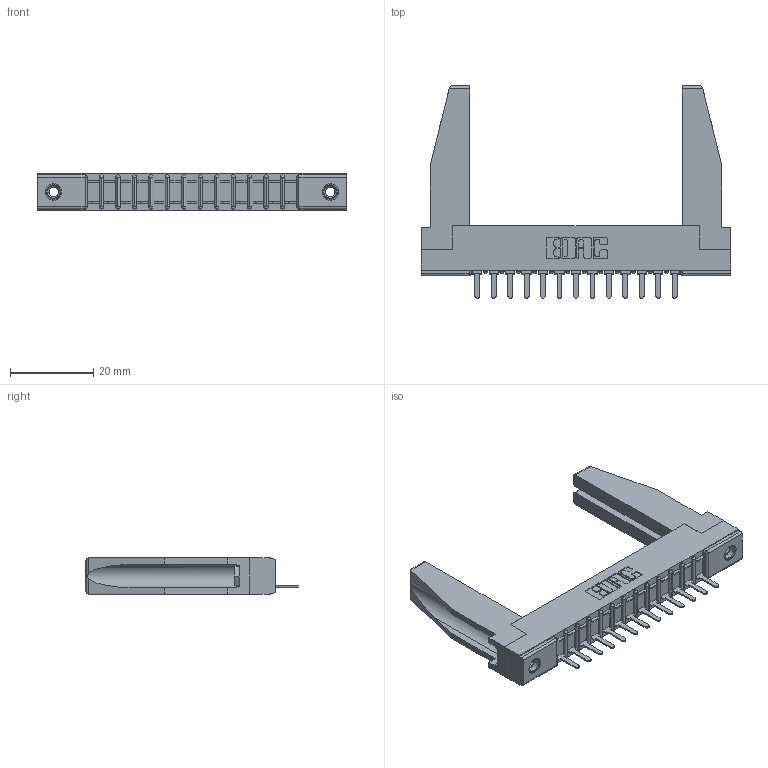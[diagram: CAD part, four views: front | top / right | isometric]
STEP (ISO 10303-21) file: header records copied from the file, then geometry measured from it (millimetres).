
FILE_DESCRIPTION (( 'STEP AP203' ), '1' );
FILE_NAME ('307-013-421-178.STEP', '2020-09-25T13:53:39', ( '' ), ( '' ), 'SwSTEP 2.0', 'SolidWorks 2020', '' );
FILE_SCHEMA (( 'CONFIG_CONTROL_DESIGN' ));
Length unit declared in the file: inch
Products named in the file (5): 307-220-078; 307-290-002_521; 307-013-421-178; 307 Part_.156 Dia Mounting Holes; 345-250-001_345-250-001-102
Assembly tree (18 placements, depth 2):
  307-013-421-178
    307 Part_.156 Dia Mounting Holes
    307-290-002_521  x13
    307-220-078  x2
    345-250-001_345-250-001-102  x2
Bounding box: 74.52 x 51.13 x 8.71 mm (x, y, z)
Volume: 8909.3 mm3; surface area: 12269.4 mm2
Topology: 18 solids, 18 shells, 1224 faces, 3669 edges, 2398 vertices
Faces by surface type: plane 739, cylinder 441, sphere 28, cone 12, torus 4
Entity records: 17877 total; most frequent: CARTESIAN_POINT 3010, ORIENTED_EDGE 2956, DIRECTION 2894, EDGE_CURVE 1478, LINE 1122, VECTOR 1122, VERTEX_POINT 960, AXIS2_PLACEMENT_3D 886
